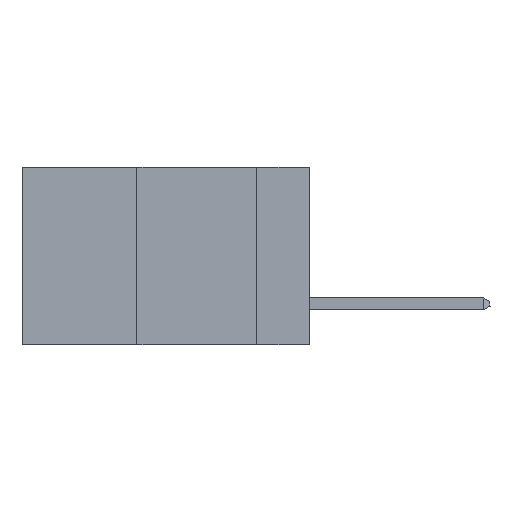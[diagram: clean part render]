
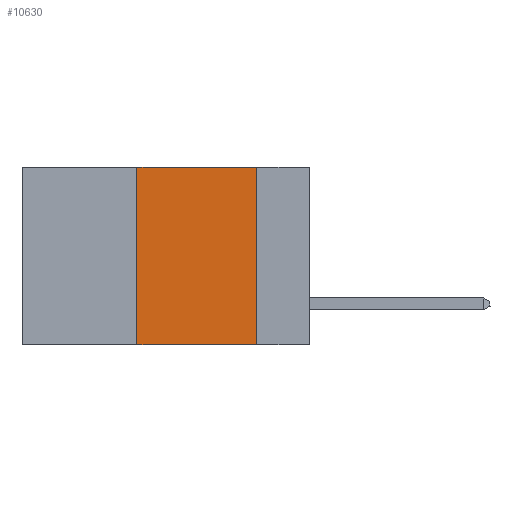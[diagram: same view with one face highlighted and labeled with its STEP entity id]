
A CAD part, left-side view. The second image highlights one B-rep face of the part: STEP entity #10630.
In plain terms, the highlighted planar face has unit normal (-1, 0, 0).
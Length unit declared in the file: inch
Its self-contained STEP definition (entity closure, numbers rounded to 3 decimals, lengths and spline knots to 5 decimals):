
#373 = DIRECTION ( 'NONE',  ( 0., 0., 1. ) ) ;
#1152 = CARTESIAN_POINT ( 'NONE',  ( 0., 0.36, -0.37 ) ) ;
#1300 = LINE ( 'NONE', #12054, #8351 ) ;
#1658 = EDGE_CURVE ( 'NONE', #5505, #11045, #9743, .T. ) ;
#1765 = DIRECTION ( 'NONE',  ( 0., -1., 0. ) ) ;
#2690 = CARTESIAN_POINT ( 'NONE',  ( 0., 0.6, 0. ) ) ;
#3232 = EDGE_CURVE ( 'NONE', #11045, #3566, #1300, .T. ) ;
#3351 = DIRECTION ( 'NONE',  ( 0., 0., -1. ) ) ;
#3398 = AXIS2_PLACEMENT_3D ( 'NONE', #2690, #3895, #12555 ) ;
#3566 = VERTEX_POINT ( 'NONE', #4032 ) ;
#3632 = EDGE_LOOP ( 'NONE', ( #11014, #5818, #6209, #9176 ) ) ;
#3895 = DIRECTION ( 'NONE',  ( 1., 0., 0. ) ) ;
#3993 = EDGE_CURVE ( 'NONE', #9254, #3566, #5116, .T. ) ;
#4032 = CARTESIAN_POINT ( 'NONE',  ( 0., 0.11, -0.37 ) ) ;
#4840 = LINE ( 'NONE', #6715, #14090 ) ;
#5116 = LINE ( 'NONE', #13534, #14962 ) ;
#5505 = VERTEX_POINT ( 'NONE', #13406 ) ;
#5818 = ORIENTED_EDGE ( 'NONE', *, *, #1658, .F. ) ;
#5823 = VECTOR ( 'NONE', #1765, 39.37008 ) ;
#6209 = ORIENTED_EDGE ( 'NONE', *, *, #11829, .F. ) ;
#6715 = CARTESIAN_POINT ( 'NONE',  ( 0., 0.36, 0. ) ) ;
#6776 = CARTESIAN_POINT ( 'NONE',  ( 0., 0.11, 0. ) ) ;
#7933 = CARTESIAN_POINT ( 'NONE',  ( 0., 0.6, 0. ) ) ;
#8351 = VECTOR ( 'NONE', #3351, 39.37008 ) ;
#9176 = ORIENTED_EDGE ( 'NONE', *, *, #3993, .T. ) ;
#9254 = VERTEX_POINT ( 'NONE', #1152 ) ;
#9743 = LINE ( 'NONE', #7933, #5823 ) ;
#10063 = PLANE ( 'NONE',  #3398 ) ;
#10630 = ADVANCED_FACE ( 'NONE', ( #14939 ), #10063, .F. ) ;
#11014 = ORIENTED_EDGE ( 'NONE', *, *, #3232, .F. ) ;
#11045 = VERTEX_POINT ( 'NONE', #6776 ) ;
#11829 = EDGE_CURVE ( 'NONE', #9254, #5505, #4840, .T. ) ;
#12054 = CARTESIAN_POINT ( 'NONE',  ( 0., 0.11, 0. ) ) ;
#12555 = DIRECTION ( 'NONE',  ( 0., 0., -1. ) ) ;
#13406 = CARTESIAN_POINT ( 'NONE',  ( 0., 0.36, 0. ) ) ;
#13534 = CARTESIAN_POINT ( 'NONE',  ( 0., 0.6, -0.37 ) ) ;
#14090 = VECTOR ( 'NONE', #373, 39.37008 ) ;
#14939 = FACE_OUTER_BOUND ( 'NONE', #3632, .T. ) ;
#14962 = VECTOR ( 'NONE', #16046, 39.37008 ) ;
#16046 = DIRECTION ( 'NONE',  ( 0., -1., 0. ) ) ;
